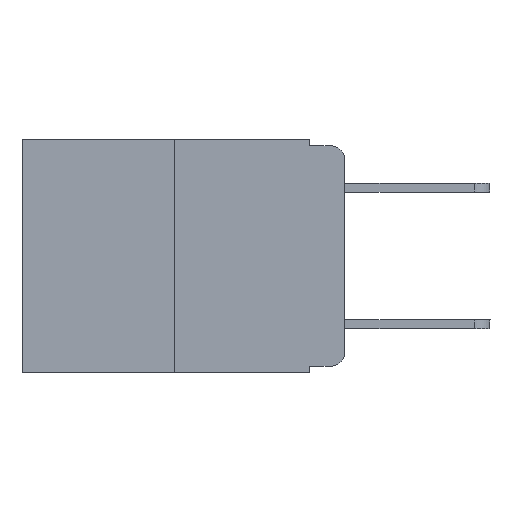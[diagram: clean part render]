
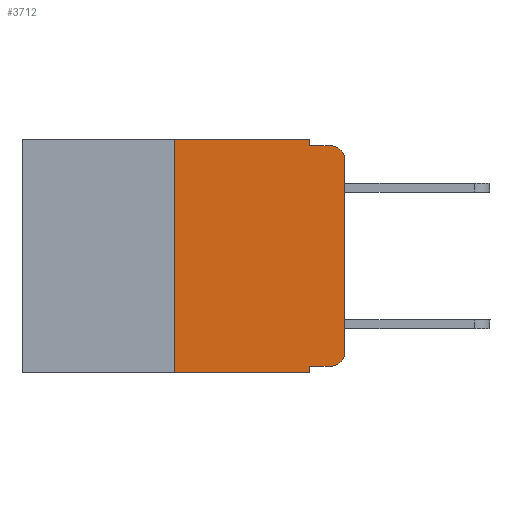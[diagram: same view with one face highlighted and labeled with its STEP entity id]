
A CAD part, left-side view. The second image highlights one B-rep face of the part: STEP entity #3712.
In plain terms, the highlighted planar face has unit normal (-1, 0, 0).
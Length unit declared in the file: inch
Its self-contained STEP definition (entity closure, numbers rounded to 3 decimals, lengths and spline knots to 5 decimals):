
#83 = CARTESIAN_POINT ( 'NONE',  ( 0., 0.051, -0.343 ) ) ;
#111 = ORIENTED_EDGE ( 'NONE', *, *, #10497, .T. ) ;
#266 = VERTEX_POINT ( 'NONE', #7155 ) ;
#389 = CARTESIAN_POINT ( 'NONE',  ( 0., 0.473, -0.343 ) ) ;
#523 = LINE ( 'NONE', #2047, #964 ) ;
#710 = EDGE_CURVE ( 'NONE', #8832, #11556, #1739, .T. ) ;
#964 = VECTOR ( 'NONE', #6600, 39.37008 ) ;
#965 = LINE ( 'NONE', #3126, #7167 ) ;
#1003 = VERTEX_POINT ( 'NONE', #83 ) ;
#1221 = EDGE_CURVE ( 'NONE', #11556, #4142, #8655, .T. ) ;
#1268 = LINE ( 'NONE', #8320, #7906 ) ;
#1334 = VERTEX_POINT ( 'NONE', #7779 ) ;
#1602 = DIRECTION ( 'NONE',  ( 0., 0., 1. ) ) ;
#1739 = CIRCLE ( 'NONE', #3137, 0.02 ) ;
#1823 = FACE_OUTER_BOUND ( 'NONE', #7552, .T. ) ;
#2047 = CARTESIAN_POINT ( 'NONE',  ( 0., 0.051, 0. ) ) ;
#2125 = CARTESIAN_POINT ( 'NONE',  ( 0., 0., -0.03 ) ) ;
#2205 = CARTESIAN_POINT ( 'NONE',  ( 0., 0., 0. ) ) ;
#2633 = DIRECTION ( 'NONE',  ( 1., 0., 0. ) ) ;
#2767 = EDGE_CURVE ( 'NONE', #266, #4585, #1268, .T. ) ;
#3089 = AXIS2_PLACEMENT_3D ( 'NONE', #7124, #2633, #7774 ) ;
#3126 = CARTESIAN_POINT ( 'NONE',  ( 0., 0.051, 0. ) ) ;
#3137 = AXIS2_PLACEMENT_3D ( 'NONE', #6829, #3310, #4249 ) ;
#3310 = DIRECTION ( 'NONE',  ( -1., 0., 0. ) ) ;
#3712 = ADVANCED_FACE ( 'NONE', ( #1823 ), #5205, .F. ) ;
#3783 = ORIENTED_EDGE ( 'NONE', *, *, #2767, .F. ) ;
#3793 = DIRECTION ( 'NONE',  ( 0., -1., 0. ) ) ;
#3921 = DIRECTION ( 'NONE',  ( 0., 0., 1. ) ) ;
#3927 = DIRECTION ( 'NONE',  ( -1., 0., 0. ) ) ;
#3998 = LINE ( 'NONE', #7147, #11606 ) ;
#4085 = DIRECTION ( 'NONE',  ( 0., -1., 0. ) ) ;
#4092 = CIRCLE ( 'NONE', #6226, 0.02 ) ;
#4142 = VERTEX_POINT ( 'NONE', #2125 ) ;
#4191 = CARTESIAN_POINT ( 'NONE',  ( 0., 0.25, 0. ) ) ;
#4249 = DIRECTION ( 'NONE',  ( 0., 0., -1. ) ) ;
#4363 = EDGE_CURVE ( 'NONE', #1334, #266, #965, .T. ) ;
#4371 = CARTESIAN_POINT ( 'NONE',  ( 0., 0.473, 0. ) ) ;
#4539 = ORIENTED_EDGE ( 'NONE', *, *, #5074, .T. ) ;
#4585 = VERTEX_POINT ( 'NONE', #11335 ) ;
#4838 = LINE ( 'NONE', #389, #5246 ) ;
#4988 = LINE ( 'NONE', #10441, #6821 ) ;
#5074 = EDGE_CURVE ( 'NONE', #4142, #4585, #4092, .T. ) ;
#5205 = PLANE ( 'NONE',  #3089 ) ;
#5246 = VECTOR ( 'NONE', #4085, 39.37008 ) ;
#5268 = VECTOR ( 'NONE', #6938, 39.37008 ) ;
#5446 = CARTESIAN_POINT ( 'NONE',  ( 0., 0.25, -0.343 ) ) ;
#5658 = EDGE_CURVE ( 'NONE', #10734, #1003, #523, .T. ) ;
#5881 = CARTESIAN_POINT ( 'NONE',  ( 0., 0.02, -0.03 ) ) ;
#5935 = DIRECTION ( 'NONE',  ( 0., -1., 0. ) ) ;
#6226 = AXIS2_PLACEMENT_3D ( 'NONE', #5881, #3927, #9388 ) ;
#6387 = ORIENTED_EDGE ( 'NONE', *, *, #1221, .T. ) ;
#6470 = ORIENTED_EDGE ( 'NONE', *, *, #710, .T. ) ;
#6600 = DIRECTION ( 'NONE',  ( 0., 0., -1. ) ) ;
#6805 = ORIENTED_EDGE ( 'NONE', *, *, #4363, .F. ) ;
#6821 = VECTOR ( 'NONE', #5935, 39.37008 ) ;
#6829 = CARTESIAN_POINT ( 'NONE',  ( 0., 0.02, -0.313 ) ) ;
#6913 = ORIENTED_EDGE ( 'NONE', *, *, #9634, .F. ) ;
#6938 = DIRECTION ( 'NONE',  ( 0., -1., 0. ) ) ;
#6947 = LINE ( 'NONE', #4371, #5268 ) ;
#6958 = VECTOR ( 'NONE', #3921, 39.37008 ) ;
#7124 = CARTESIAN_POINT ( 'NONE',  ( 0., 0.473, 0. ) ) ;
#7147 = CARTESIAN_POINT ( 'NONE',  ( 0., 0.25, 0. ) ) ;
#7155 = CARTESIAN_POINT ( 'NONE',  ( 0., 0.051, -0.01 ) ) ;
#7167 = VECTOR ( 'NONE', #7503, 39.37008 ) ;
#7503 = DIRECTION ( 'NONE',  ( 0., 0., -1. ) ) ;
#7552 = EDGE_LOOP ( 'NONE', ( #6387, #4539, #3783, #6805, #6913, #8289, #111, #9779, #7628, #6470 ) ) ;
#7628 = ORIENTED_EDGE ( 'NONE', *, *, #9493, .T. ) ;
#7774 = DIRECTION ( 'NONE',  ( 0., 0., -1. ) ) ;
#7779 = CARTESIAN_POINT ( 'NONE',  ( 0., 0.051, 0. ) ) ;
#7906 = VECTOR ( 'NONE', #3793, 39.37008 ) ;
#7977 = VERTEX_POINT ( 'NONE', #4191 ) ;
#8289 = ORIENTED_EDGE ( 'NONE', *, *, #10036, .F. ) ;
#8320 = CARTESIAN_POINT ( 'NONE',  ( 0., 0.051, -0.01 ) ) ;
#8421 = CARTESIAN_POINT ( 'NONE',  ( 0., 0., -0.313 ) ) ;
#8582 = VERTEX_POINT ( 'NONE', #5446 ) ;
#8655 = LINE ( 'NONE', #2205, #6958 ) ;
#8832 = VERTEX_POINT ( 'NONE', #10673 ) ;
#9388 = DIRECTION ( 'NONE',  ( 0., 0., -1. ) ) ;
#9493 = EDGE_CURVE ( 'NONE', #10734, #8832, #4988, .T. ) ;
#9634 = EDGE_CURVE ( 'NONE', #7977, #1334, #6947, .T. ) ;
#9779 = ORIENTED_EDGE ( 'NONE', *, *, #5658, .F. ) ;
#10036 = EDGE_CURVE ( 'NONE', #8582, #7977, #3998, .T. ) ;
#10441 = CARTESIAN_POINT ( 'NONE',  ( 0., 0.051, -0.333 ) ) ;
#10497 = EDGE_CURVE ( 'NONE', #8582, #1003, #4838, .T. ) ;
#10647 = CARTESIAN_POINT ( 'NONE',  ( 0., 0.051, -0.333 ) ) ;
#10673 = CARTESIAN_POINT ( 'NONE',  ( 0., 0.02, -0.333 ) ) ;
#10734 = VERTEX_POINT ( 'NONE', #10647 ) ;
#11335 = CARTESIAN_POINT ( 'NONE',  ( 0., 0.02, -0.01 ) ) ;
#11556 = VERTEX_POINT ( 'NONE', #8421 ) ;
#11606 = VECTOR ( 'NONE', #1602, 39.37008 ) ;
